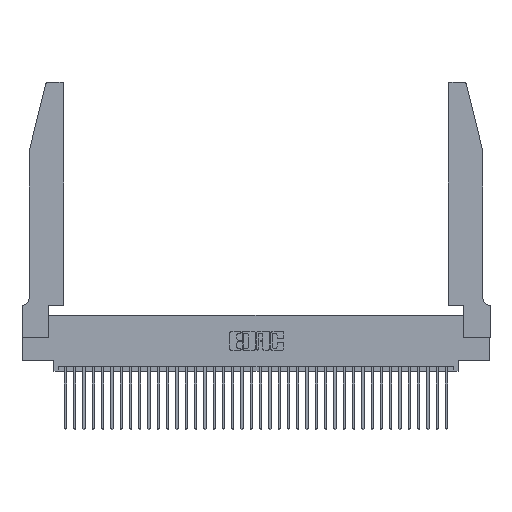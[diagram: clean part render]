
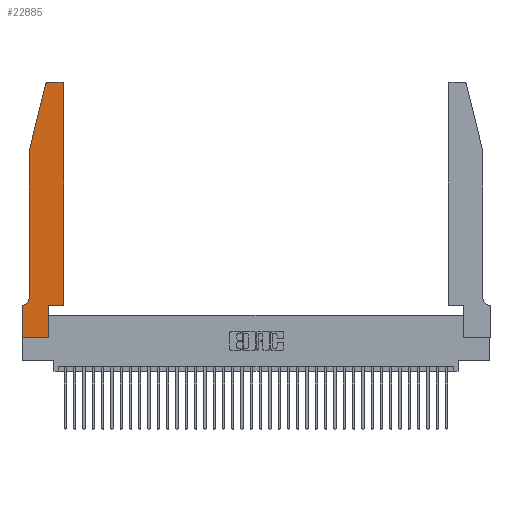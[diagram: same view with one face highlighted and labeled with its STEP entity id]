
A CAD part, top view. The second image highlights one B-rep face of the part: STEP entity #22885.
In plain terms, the highlighted planar face has unit normal (0, 0, 1).
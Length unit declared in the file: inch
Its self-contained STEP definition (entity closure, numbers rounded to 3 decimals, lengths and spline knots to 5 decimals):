
#153 = CARTESIAN_POINT ( 'NONE',  ( 0.4205, 2.72, 0.37 ) ) ;
#339 = CARTESIAN_POINT ( 'NONE',  ( 0.2605, 2.75, 0.37 ) ) ;
#1019 = ORIENTED_EDGE ( 'NONE', *, *, #11333, .T. ) ;
#1280 = ORIENTED_EDGE ( 'NONE', *, *, #5635, .T. ) ;
#1629 = LINE ( 'NONE', #36809, #17506 ) ;
#1846 = EDGE_CURVE ( 'NONE', #33952, #16267, #30323, .T. ) ;
#2772 = VERTEX_POINT ( 'NONE', #19839 ) ;
#2900 = CARTESIAN_POINT ( 'NONE',  ( 0.0755, 2., 0.37 ) ) ;
#3190 = DIRECTION ( 'NONE',  ( 1., 0., 0. ) ) ;
#4063 = ORIENTED_EDGE ( 'NONE', *, *, #5176, .T. ) ;
#4681 = CARTESIAN_POINT ( 'NONE',  ( 0.4505, 0.35, 0.37 ) ) ;
#4754 = VECTOR ( 'NONE', #20283, 39.37008 ) ;
#5176 = EDGE_CURVE ( 'NONE', #35281, #21252, #18712, .T. ) ;
#5233 = CARTESIAN_POINT ( 'NONE',  ( 0.0755, 2., 0.37 ) ) ;
#5239 = AXIS2_PLACEMENT_3D ( 'NONE', #153, #20914, #3190 ) ;
#5635 = EDGE_CURVE ( 'NONE', #21252, #32729, #13659, .T. ) ;
#5740 = ORIENTED_EDGE ( 'NONE', *, *, #20382, .T. ) ;
#6256 = CARTESIAN_POINT ( 'NONE',  ( 0.284, 2.72, 0.37 ) ) ;
#7078 = AXIS2_PLACEMENT_3D ( 'NONE', #6256, #26700, #9267 ) ;
#8052 = ORIENTED_EDGE ( 'NONE', *, *, #22034, .T. ) ;
#8113 = CARTESIAN_POINT ( 'NONE',  ( 0.2865, 0.35, 0.37 ) ) ;
#8363 = DIRECTION ( 'NONE',  ( 0., 0., -1. ) ) ;
#8601 = ORIENTED_EDGE ( 'NONE', *, *, #1846, .T. ) ;
#9014 = EDGE_CURVE ( 'NONE', #17196, #27051, #1629, .T. ) ;
#9267 = DIRECTION ( 'NONE',  ( 1., 0., 0. ) ) ;
#9657 = LINE ( 'NONE', #4681, #24279 ) ;
#9915 = ORIENTED_EDGE ( 'NONE', *, *, #9014, .T. ) ;
#9935 = FACE_OUTER_BOUND ( 'NONE', #31710, .T. ) ;
#10006 = CARTESIAN_POINT ( 'NONE',  ( 0., 0., 0.37 ) ) ;
#11054 = PLANE ( 'NONE',  #16110 ) ;
#11333 = EDGE_CURVE ( 'NONE', #16267, #35281, #36713, .T. ) ;
#11722 = VERTEX_POINT ( 'NONE', #8113 ) ;
#11958 = VECTOR ( 'NONE', #30246, 39.37008 ) ;
#12500 = VERTEX_POINT ( 'NONE', #37438 ) ;
#13374 = ORIENTED_EDGE ( 'NONE', *, *, #33895, .T. ) ;
#13659 = LINE ( 'NONE', #34569, #4754 ) ;
#13905 = DIRECTION ( 'NONE',  ( -1., 0., 0. ) ) ;
#14455 = CARTESIAN_POINT ( 'NONE',  ( 0., 0.35, 0.37 ) ) ;
#14514 = CARTESIAN_POINT ( 'NONE',  ( 0.4505, 2.72, 0.37 ) ) ;
#16110 = AXIS2_PLACEMENT_3D ( 'NONE', #31247, #16961, #37060 ) ;
#16267 = VERTEX_POINT ( 'NONE', #30351 ) ;
#16676 = DIRECTION ( 'NONE',  ( 1., 0., 0. ) ) ;
#16961 = DIRECTION ( 'NONE',  ( 0., 0., 1. ) ) ;
#17196 = VERTEX_POINT ( 'NONE', #34601 ) ;
#17506 = VECTOR ( 'NONE', #13905, 39.37008 ) ;
#18037 = VERTEX_POINT ( 'NONE', #23226 ) ;
#18694 = LINE ( 'NONE', #5233, #25406 ) ;
#18712 = CIRCLE ( 'NONE', #7078, 0.03 ) ;
#18995 = VECTOR ( 'NONE', #36141, 39.37008 ) ;
#19000 = ORIENTED_EDGE ( 'NONE', *, *, #23631, .T. ) ;
#19839 = CARTESIAN_POINT ( 'NONE',  ( 0.0755, 0.42, 0.37 ) ) ;
#20087 = DIRECTION ( 'NONE',  ( 0., -1., 0. ) ) ;
#20283 = DIRECTION ( 'NONE',  ( -0.239, -0.971, 0. ) ) ;
#20382 = EDGE_CURVE ( 'NONE', #11722, #12500, #9657, .T. ) ;
#20686 = VERTEX_POINT ( 'NONE', #26568 ) ;
#20914 = DIRECTION ( 'NONE',  ( 0., 0., 1. ) ) ;
#20981 = EDGE_CURVE ( 'NONE', #18037, #20686, #34070, .T. ) ;
#21252 = VERTEX_POINT ( 'NONE', #34524 ) ;
#21559 = DIRECTION ( 'NONE',  ( 0., 1., 0. ) ) ;
#22034 = EDGE_CURVE ( 'NONE', #12500, #33952, #29480, .T. ) ;
#22677 = ORIENTED_EDGE ( 'NONE', *, *, #20981, .T. ) ;
#22717 = LINE ( 'NONE', #30378, #37104 ) ;
#22885 = ADVANCED_FACE ( 'NONE', ( #9935 ), #11054, .T. ) ;
#23226 = CARTESIAN_POINT ( 'NONE',  ( 0., 0., 0.37 ) ) ;
#23631 = EDGE_CURVE ( 'NONE', #2772, #17196, #30704, .T. ) ;
#24043 = ORIENTED_EDGE ( 'NONE', *, *, #29301, .T. ) ;
#24279 = VECTOR ( 'NONE', #16676, 39.37008 ) ;
#24322 = AXIS2_PLACEMENT_3D ( 'NONE', #25822, #8363, #28710 ) ;
#24779 = DIRECTION ( 'NONE',  ( 0., 1., 0. ) ) ;
#25406 = VECTOR ( 'NONE', #20087, 39.37008 ) ;
#25822 = CARTESIAN_POINT ( 'NONE',  ( 0.0055, 0.42, 0.37 ) ) ;
#26568 = CARTESIAN_POINT ( 'NONE',  ( 0.2865, 0., 0.37 ) ) ;
#26700 = DIRECTION ( 'NONE',  ( 0., 0., 1. ) ) ;
#27051 = VERTEX_POINT ( 'NONE', #14455 ) ;
#27278 = VECTOR ( 'NONE', #29852, 39.37008 ) ;
#27487 = CARTESIAN_POINT ( 'NONE',  ( 0., 0., 0.37 ) ) ;
#27505 = LINE ( 'NONE', #27487, #18995 ) ;
#28596 = VECTOR ( 'NONE', #21559, 39.37008 ) ;
#28710 = DIRECTION ( 'NONE',  ( -1., 0., 0. ) ) ;
#29301 = EDGE_CURVE ( 'NONE', #20686, #11722, #22717, .T. ) ;
#29480 = LINE ( 'NONE', #33075, #28596 ) ;
#29852 = DIRECTION ( 'NONE',  ( -1., 0., 0. ) ) ;
#30246 = DIRECTION ( 'NONE',  ( 1., 0., 0. ) ) ;
#30323 = CIRCLE ( 'NONE', #5239, 0.03 ) ;
#30351 = CARTESIAN_POINT ( 'NONE',  ( 0.4205, 2.75, 0.37 ) ) ;
#30378 = CARTESIAN_POINT ( 'NONE',  ( 0.2865, 0.35, 0.37 ) ) ;
#30704 = CIRCLE ( 'NONE', #24322, 0.07 ) ;
#31247 = CARTESIAN_POINT ( 'NONE',  ( 0., 0.35, 0.37 ) ) ;
#31710 = EDGE_LOOP ( 'NONE', ( #1019, #4063, #1280, #13374, #19000, #9915, #34814, #22677, #24043, #5740, #8052, #8601 ) ) ;
#32729 = VERTEX_POINT ( 'NONE', #2900 ) ;
#33075 = CARTESIAN_POINT ( 'NONE',  ( 0.4505, 0.35, 0.37 ) ) ;
#33523 = CARTESIAN_POINT ( 'NONE',  ( 0.284, 2.75, 0.37 ) ) ;
#33895 = EDGE_CURVE ( 'NONE', #32729, #2772, #18694, .T. ) ;
#33952 = VERTEX_POINT ( 'NONE', #14514 ) ;
#34070 = LINE ( 'NONE', #10006, #11958 ) ;
#34524 = CARTESIAN_POINT ( 'NONE',  ( 0.25487, 2.72718, 0.37 ) ) ;
#34569 = CARTESIAN_POINT ( 'NONE',  ( 0.0755, 2., 0.37 ) ) ;
#34601 = CARTESIAN_POINT ( 'NONE',  ( 0.0055, 0.35, 0.37 ) ) ;
#34814 = ORIENTED_EDGE ( 'NONE', *, *, #35889, .T. ) ;
#35281 = VERTEX_POINT ( 'NONE', #33523 ) ;
#35889 = EDGE_CURVE ( 'NONE', #27051, #18037, #27505, .T. ) ;
#36141 = DIRECTION ( 'NONE',  ( 0., -1., 0. ) ) ;
#36713 = LINE ( 'NONE', #339, #27278 ) ;
#36809 = CARTESIAN_POINT ( 'NONE',  ( 0.0755, 0.35, 0.37 ) ) ;
#37060 = DIRECTION ( 'NONE',  ( 1., 0., 0. ) ) ;
#37104 = VECTOR ( 'NONE', #24779, 39.37008 ) ;
#37438 = CARTESIAN_POINT ( 'NONE',  ( 0.4505, 0.35, 0.37 ) ) ;
